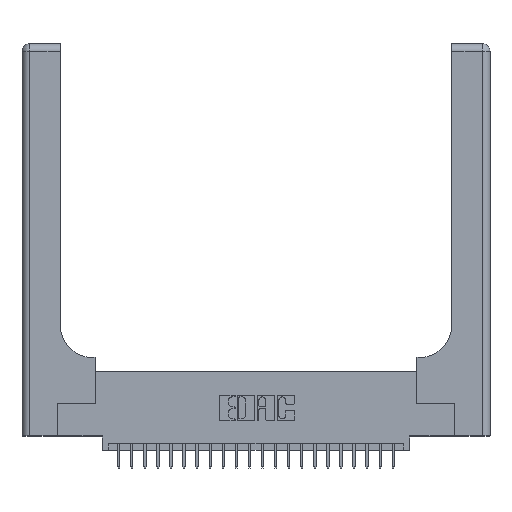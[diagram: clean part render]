
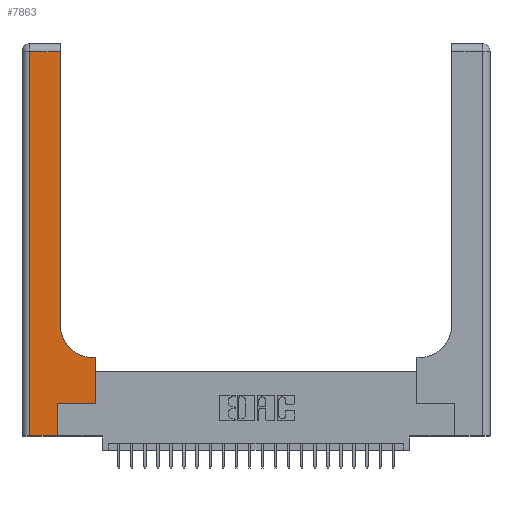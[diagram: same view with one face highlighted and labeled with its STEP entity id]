
A CAD part, top view. The second image highlights one B-rep face of the part: STEP entity #7863.
In plain terms, the highlighted planar face has unit normal (0, 0, 1).
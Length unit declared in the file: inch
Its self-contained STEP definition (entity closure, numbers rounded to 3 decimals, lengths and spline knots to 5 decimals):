
#55 = ORIENTED_EDGE ( 'NONE', *, *, #19095, .T. ) ;
#95 = EDGE_CURVE ( 'NONE', #15142, #21993, #19224, .T. ) ;
#346 = ORIENTED_EDGE ( 'NONE', *, *, #10486, .T. ) ;
#1236 = PLANE ( 'NONE',  #6706 ) ;
#1557 = LINE ( 'NONE', #15604, #2778 ) ;
#2662 = CARTESIAN_POINT ( 'NONE',  ( 0.5585, 0.6, 0.37 ) ) ;
#2702 = ORIENTED_EDGE ( 'NONE', *, *, #95, .T. ) ;
#2778 = VECTOR ( 'NONE', #13208, 39.37008 ) ;
#3018 = CIRCLE ( 'NONE', #20590, 0.25 ) ;
#4254 = LINE ( 'NONE', #21654, #21533 ) ;
#4873 = EDGE_CURVE ( 'NONE', #5334, #10853, #25278, .T. ) ;
#5334 = VERTEX_POINT ( 'NONE', #9458 ) ;
#5579 = CARTESIAN_POINT ( 'NONE',  ( 0., 2.94, 0.37 ) ) ;
#5715 = VERTEX_POINT ( 'NONE', #7673 ) ;
#5765 = VECTOR ( 'NONE', #19477, 39.37008 ) ;
#6318 = ORIENTED_EDGE ( 'NONE', *, *, #7635, .T. ) ;
#6706 = AXIS2_PLACEMENT_3D ( 'NONE', #17095, #13748, #13276 ) ;
#6907 = LINE ( 'NONE', #24197, #15156 ) ;
#7388 = DIRECTION ( 'NONE',  ( 0., 1., 0. ) ) ;
#7635 = EDGE_CURVE ( 'NONE', #13804, #19241, #12145, .T. ) ;
#7673 = CARTESIAN_POINT ( 'NONE',  ( 0.5585, 0.25, 0.37 ) ) ;
#7728 = DIRECTION ( 'NONE',  ( -1., 0., 0. ) ) ;
#7863 = ADVANCED_FACE ( 'NONE', ( #16853 ), #1236, .F. ) ;
#7986 = CARTESIAN_POINT ( 'NONE',  ( 0.5415, 0.6, 0.37 ) ) ;
#9138 = LINE ( 'NONE', #10533, #13364 ) ;
#9458 = CARTESIAN_POINT ( 'NONE',  ( 0.2915, 2.94, 0.37 ) ) ;
#9848 = VECTOR ( 'NONE', #7728, 39.37008 ) ;
#10486 = EDGE_CURVE ( 'NONE', #19241, #22159, #15132, .T. ) ;
#10533 = CARTESIAN_POINT ( 'NONE',  ( 0.5585, 0.25, 0.37 ) ) ;
#10563 = DIRECTION ( 'NONE',  ( 0., 1., 0. ) ) ;
#10727 = EDGE_CURVE ( 'NONE', #21993, #13708, #3018, .T. ) ;
#10853 = VERTEX_POINT ( 'NONE', #24388 ) ;
#11048 = ORIENTED_EDGE ( 'NONE', *, *, #10727, .T. ) ;
#11898 = CARTESIAN_POINT ( 'NONE',  ( 0., 0., 0.37 ) ) ;
#11981 = VECTOR ( 'NONE', #21509, 39.37008 ) ;
#12145 = LINE ( 'NONE', #11898, #11981 ) ;
#12474 = ORIENTED_EDGE ( 'NONE', *, *, #20777, .T. ) ;
#12900 = CARTESIAN_POINT ( 'NONE',  ( 0.2915, 0.85, 0.37 ) ) ;
#13208 = DIRECTION ( 'NONE',  ( 1., 0., 0. ) ) ;
#13276 = DIRECTION ( 'NONE',  ( -1., 0., 0. ) ) ;
#13348 = CARTESIAN_POINT ( 'NONE',  ( 0.2915, 0.6, 0.37 ) ) ;
#13364 = VECTOR ( 'NONE', #22380, 39.37008 ) ;
#13708 = VERTEX_POINT ( 'NONE', #12900 ) ;
#13748 = DIRECTION ( 'NONE',  ( 0., 0., -1. ) ) ;
#13804 = VERTEX_POINT ( 'NONE', #19035 ) ;
#14527 = EDGE_CURVE ( 'NONE', #5715, #15142, #9138, .T. ) ;
#15132 = LINE ( 'NONE', #17055, #22282 ) ;
#15142 = VERTEX_POINT ( 'NONE', #2662 ) ;
#15156 = VECTOR ( 'NONE', #10563, 39.37008 ) ;
#15311 = ORIENTED_EDGE ( 'NONE', *, *, #14527, .T. ) ;
#15467 = ORIENTED_EDGE ( 'NONE', *, *, #4873, .T. ) ;
#15604 = CARTESIAN_POINT ( 'NONE',  ( 0.269, 0.25, 0.37 ) ) ;
#15848 = DIRECTION ( 'NONE',  ( 0., -1., 0. ) ) ;
#16138 = DIRECTION ( 'NONE',  ( 1., 0., 0. ) ) ;
#16476 = CARTESIAN_POINT ( 'NONE',  ( 0.269, 0., 0.37 ) ) ;
#16853 = FACE_OUTER_BOUND ( 'NONE', #19793, .T. ) ;
#17055 = CARTESIAN_POINT ( 'NONE',  ( 0.269, 0., 0.37 ) ) ;
#17095 = CARTESIAN_POINT ( 'NONE',  ( 0., 3., 0.37 ) ) ;
#17641 = ORIENTED_EDGE ( 'NONE', *, *, #24417, .T. ) ;
#17809 = CARTESIAN_POINT ( 'NONE',  ( 0.269, 0.25, 0.37 ) ) ;
#19035 = CARTESIAN_POINT ( 'NONE',  ( 0.06, 0., 0.37 ) ) ;
#19095 = EDGE_CURVE ( 'NONE', #10853, #13804, #4254, .T. ) ;
#19224 = LINE ( 'NONE', #13348, #5765 ) ;
#19241 = VERTEX_POINT ( 'NONE', #16476 ) ;
#19477 = DIRECTION ( 'NONE',  ( -1., 0., 0. ) ) ;
#19793 = EDGE_LOOP ( 'NONE', ( #17641, #15467, #55, #6318, #346, #12474, #15311, #2702, #11048 ) ) ;
#19866 = DIRECTION ( 'NONE',  ( 0., 0., -1. ) ) ;
#20590 = AXIS2_PLACEMENT_3D ( 'NONE', #21830, #19866, #16138 ) ;
#20777 = EDGE_CURVE ( 'NONE', #22159, #5715, #1557, .T. ) ;
#21509 = DIRECTION ( 'NONE',  ( 1., 0., 0. ) ) ;
#21533 = VECTOR ( 'NONE', #15848, 39.37008 ) ;
#21654 = CARTESIAN_POINT ( 'NONE',  ( 0.06, 3., 0.37 ) ) ;
#21830 = CARTESIAN_POINT ( 'NONE',  ( 0.5415, 0.85, 0.37 ) ) ;
#21993 = VERTEX_POINT ( 'NONE', #7986 ) ;
#22159 = VERTEX_POINT ( 'NONE', #17809 ) ;
#22282 = VECTOR ( 'NONE', #7388, 39.37008 ) ;
#22380 = DIRECTION ( 'NONE',  ( 0., 1., 0. ) ) ;
#24197 = CARTESIAN_POINT ( 'NONE',  ( 0.2915, 3., 0.37 ) ) ;
#24388 = CARTESIAN_POINT ( 'NONE',  ( 0.06, 2.94, 0.37 ) ) ;
#24417 = EDGE_CURVE ( 'NONE', #13708, #5334, #6907, .T. ) ;
#25278 = LINE ( 'NONE', #5579, #9848 ) ;
